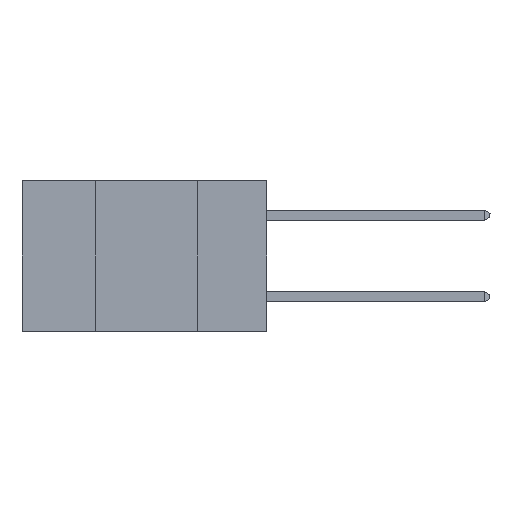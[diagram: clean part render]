
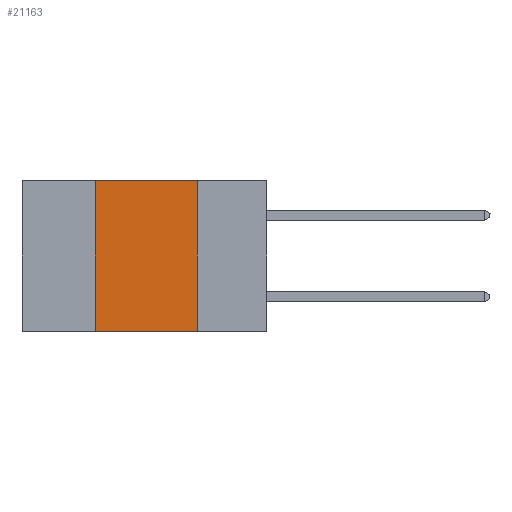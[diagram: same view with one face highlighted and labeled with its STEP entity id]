
A CAD part, left-side view. The second image highlights one B-rep face of the part: STEP entity #21163.
In plain terms, the highlighted planar face has unit normal (-1, 0, 0).
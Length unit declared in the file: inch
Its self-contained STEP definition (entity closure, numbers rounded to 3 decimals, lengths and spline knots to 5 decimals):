
#445 = ORIENTED_EDGE ( 'NONE', *, *, #8128, .F. ) ;
#918 = VECTOR ( 'NONE', #2120, 39.37008 ) ;
#2120 = DIRECTION ( 'NONE',  ( 0., -1., 0. ) ) ;
#2994 = FACE_OUTER_BOUND ( 'NONE', #12632, .T. ) ;
#3347 = EDGE_CURVE ( 'NONE', #17433, #13709, #10616, .T. ) ;
#4741 = DIRECTION ( 'NONE',  ( 0., -1., 0. ) ) ;
#4790 = LINE ( 'NONE', #5370, #918 ) ;
#5238 = CARTESIAN_POINT ( 'NONE',  ( 0., 0.6, 0. ) ) ;
#5370 = CARTESIAN_POINT ( 'NONE',  ( 0., 0.6, 0. ) ) ;
#6056 = CARTESIAN_POINT ( 'NONE',  ( 0., 0.6, -0.37 ) ) ;
#7096 = EDGE_CURVE ( 'NONE', #17433, #8247, #15736, .T. ) ;
#7552 = ORIENTED_EDGE ( 'NONE', *, *, #3347, .T. ) ;
#7988 = CARTESIAN_POINT ( 'NONE',  ( 0., 0.17, -0.37 ) ) ;
#8128 = EDGE_CURVE ( 'NONE', #8247, #19475, #4790, .T. ) ;
#8247 = VERTEX_POINT ( 'NONE', #13483 ) ;
#8799 = DIRECTION ( 'NONE',  ( 0., 0., 1. ) ) ;
#8984 = CARTESIAN_POINT ( 'NONE',  ( 0., 0.17, 0. ) ) ;
#9351 = CARTESIAN_POINT ( 'NONE',  ( 0., 0.42, 0. ) ) ;
#10017 = ORIENTED_EDGE ( 'NONE', *, *, #7096, .F. ) ;
#10616 = LINE ( 'NONE', #6056, #19150 ) ;
#12282 = DIRECTION ( 'NONE',  ( 0., 0., -1. ) ) ;
#12329 = CARTESIAN_POINT ( 'NONE',  ( 0., 0.17, 0. ) ) ;
#12632 = EDGE_LOOP ( 'NONE', ( #17528, #445, #10017, #7552 ) ) ;
#13483 = CARTESIAN_POINT ( 'NONE',  ( 0., 0.42, 0. ) ) ;
#13709 = VERTEX_POINT ( 'NONE', #7988 ) ;
#15143 = DIRECTION ( 'NONE',  ( 0., 0., -1. ) ) ;
#15378 = EDGE_CURVE ( 'NONE', #19475, #13709, #17455, .T. ) ;
#15736 = LINE ( 'NONE', #9351, #20674 ) ;
#16178 = CARTESIAN_POINT ( 'NONE',  ( 0., 0.42, -0.37 ) ) ;
#17433 = VERTEX_POINT ( 'NONE', #16178 ) ;
#17455 = LINE ( 'NONE', #8984, #18478 ) ;
#17528 = ORIENTED_EDGE ( 'NONE', *, *, #15378, .F. ) ;
#18380 = AXIS2_PLACEMENT_3D ( 'NONE', #5238, #18794, #15143 ) ;
#18478 = VECTOR ( 'NONE', #12282, 39.37008 ) ;
#18649 = PLANE ( 'NONE',  #18380 ) ;
#18794 = DIRECTION ( 'NONE',  ( 1., 0., 0. ) ) ;
#19150 = VECTOR ( 'NONE', #4741, 39.37008 ) ;
#19475 = VERTEX_POINT ( 'NONE', #12329 ) ;
#20674 = VECTOR ( 'NONE', #8799, 39.37008 ) ;
#21163 = ADVANCED_FACE ( 'NONE', ( #2994 ), #18649, .F. ) ;
